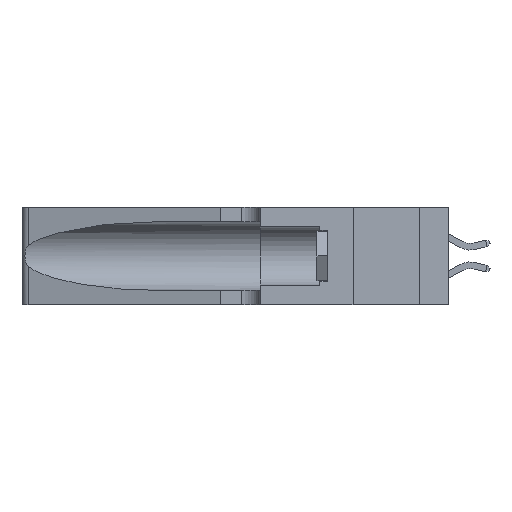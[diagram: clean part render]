
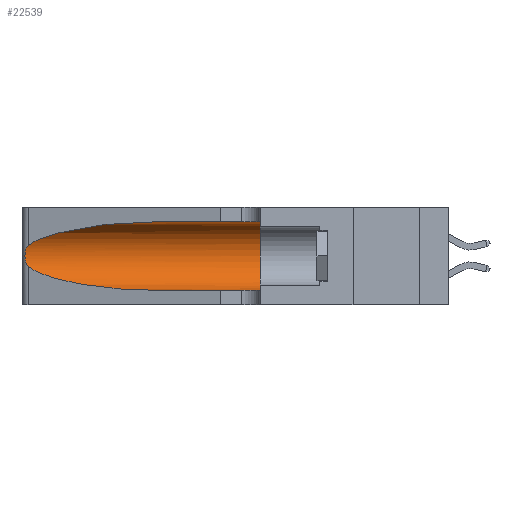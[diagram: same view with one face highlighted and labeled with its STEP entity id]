
A CAD part, left-side view. The second image highlights one B-rep face of the part: STEP entity #22539.
In plain terms, the highlighted cylindrical face has radius 3.308 mm (diameter 6.617 mm), a partial arc.
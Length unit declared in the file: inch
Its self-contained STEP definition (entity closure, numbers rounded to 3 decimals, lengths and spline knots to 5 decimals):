
#822 = AXIS2_PLACEMENT_3D ( 'NONE', #7146, #13845, #24084 ) ;
#1048 = DIRECTION ( 'NONE',  ( 0., -1., 0. ) ) ;
#2286 = CARTESIAN_POINT ( 'NONE',  ( 0.25555, 1.22994, 0.2215 ) ) ;
#2435 = CARTESIAN_POINT ( 'NONE',  ( 0.25854, 1.2359, 0.20912 ) ) ;
#2937 = CARTESIAN_POINT ( 'NONE',  ( 0.1305, 1.61858, 0.31525 ) ) ;
#3580 = VERTEX_POINT ( 'NONE', #40791 ) ;
#3627 = CARTESIAN_POINT ( 'NONE',  ( 0.1305, 0.72297, 0.05475 ) ) ;
#3670 = AXIS2_PLACEMENT_3D ( 'NONE', #38899, #18575, #42254 ) ;
#3993 = EDGE_CURVE ( 'NONE', #22033, #3580, #9045, .T. ) ;
#4248 = VERTEX_POINT ( 'NONE', #3627 ) ;
#5766 =( BOUNDED_CURVE ( )  B_SPLINE_CURVE ( 3, ( #12534, #26208, #9281, #33033 ),
 .UNSPECIFIED., .F., .F. ) 
 B_SPLINE_CURVE_WITH_KNOTS ( ( 4, 4 ),
 ( 3.44316, 4.71239 ),
 .UNSPECIFIED. ) 
 CURVE ( )  GEOMETRIC_REPRESENTATION_ITEM ( )  RATIONAL_B_SPLINE_CURVE ( ( 1., 0.87, 0.87, 1. ) ) 
 REPRESENTATION_ITEM ( '' )  );
#5879 = CARTESIAN_POINT ( 'NONE',  ( 0.26075, 1.23896, 0.19203 ) ) ;
#6364 = DIRECTION ( 'NONE',  ( 0., -1., 0. ) ) ;
#7146 = CARTESIAN_POINT ( 'NONE',  ( 0.1305, 1.61858, 0.185 ) ) ;
#7447 = CIRCLE ( 'NONE', #3670, 0.13025 ) ;
#7490 = ORIENTED_EDGE ( 'NONE', *, *, #11694, .F. ) ;
#7576 = CYLINDRICAL_SURFACE ( 'NONE', #822, 0.13025 ) ;
#8862 = CARTESIAN_POINT ( 'NONE',  ( 0.1305, 0.35, 0.05475 ) ) ;
#9045 = B_SPLINE_CURVE_WITH_KNOTS ( 'NONE', 3,
 ( #36313, #2286, #43065, #22806, #2435, #26228, #5879, #29645, #9307, #33057, #12716, #36456, #16118, #39839 ),
 .UNSPECIFIED., .F., .F.,
 ( 4, 2, 2, 2, 2, 2, 4 ),
 ( 0., 0.00027, 0.00053, 0.00107, 0.0016, 0.00187, 0.00214 ),
 .UNSPECIFIED. ) ;
#9281 = CARTESIAN_POINT ( 'NONE',  ( 0.18966, 0.96281, 0.05475 ) ) ;
#9293 = CARTESIAN_POINT ( 'NONE',  ( 0.18966, 0.96281, 0.31525 ) ) ;
#9307 = CARTESIAN_POINT ( 'NONE',  ( 0.26017, 1.23833, 0.17102 ) ) ;
#11694 = EDGE_CURVE ( 'NONE', #39162, #39043, #23999, .T. ) ;
#11950 = ORIENTED_EDGE ( 'NONE', *, *, #17912, .T. ) ;
#12534 = CARTESIAN_POINT ( 'NONE',  ( 0.25487, 1.22718, 0.14631 ) ) ;
#12716 = CARTESIAN_POINT ( 'NONE',  ( 0.25789, 1.23486, 0.15765 ) ) ;
#13516 = ORIENTED_EDGE ( 'NONE', *, *, #3993, .T. ) ;
#13845 = DIRECTION ( 'NONE',  ( 0., -1., 0. ) ) ;
#14814 = EDGE_CURVE ( 'NONE', #39162, #22033, #21548, .T. ) ;
#16118 = CARTESIAN_POINT ( 'NONE',  ( 0.25555, 1.22993, 0.14849 ) ) ;
#16540 = EDGE_CURVE ( 'NONE', #39043, #33109, #7447, .T. ) ;
#17296 = LINE ( 'NONE', #41724, #34305 ) ;
#17853 = EDGE_LOOP ( 'NONE', ( #41080, #13516, #11950, #31107, #41205, #7490 ) ) ;
#17912 = EDGE_CURVE ( 'NONE', #3580, #4248, #5766, .T. ) ;
#18575 = DIRECTION ( 'NONE',  ( 0., 1., 0. ) ) ;
#19530 = CARTESIAN_POINT ( 'NONE',  ( 0.25487, 1.22718, 0.22369 ) ) ;
#21548 =( BOUNDED_CURVE ( )  B_SPLINE_CURVE ( 3, ( #36437, #9293, #39831, #19530 ),
 .UNSPECIFIED., .F., .F. ) 
 B_SPLINE_CURVE_WITH_KNOTS ( ( 4, 4 ),
 ( 1.5708, 2.84003 ),
 .UNSPECIFIED. ) 
 CURVE ( )  GEOMETRIC_REPRESENTATION_ITEM ( )  RATIONAL_B_SPLINE_CURVE ( ( 1., 0.87, 0.87, 1. ) ) 
 REPRESENTATION_ITEM ( '' )  );
#21874 = CARTESIAN_POINT ( 'NONE',  ( 0.1305, 0.35, 0.31525 ) ) ;
#22033 = VERTEX_POINT ( 'NONE', #38663 ) ;
#22539 = ADVANCED_FACE ( 'NONE', ( #34670 ), #7576, .F. ) ;
#22806 = CARTESIAN_POINT ( 'NONE',  ( 0.25787, 1.23484, 0.2124 ) ) ;
#23999 = LINE ( 'NONE', #2937, #40957 ) ;
#24084 = DIRECTION ( 'NONE',  ( 0., 0., -1. ) ) ;
#26208 = CARTESIAN_POINT ( 'NONE',  ( 0.2373, 1.15595, 0.08982 ) ) ;
#26228 = CARTESIAN_POINT ( 'NONE',  ( 0.26018, 1.23835, 0.19895 ) ) ;
#29645 = CARTESIAN_POINT ( 'NONE',  ( 0.26075, 1.23896, 0.178 ) ) ;
#31107 = ORIENTED_EDGE ( 'NONE', *, *, #38966, .T. ) ;
#33033 = CARTESIAN_POINT ( 'NONE',  ( 0.1305, 0.72297, 0.05475 ) ) ;
#33057 = CARTESIAN_POINT ( 'NONE',  ( 0.25856, 1.23593, 0.16098 ) ) ;
#33109 = VERTEX_POINT ( 'NONE', #8862 ) ;
#34305 = VECTOR ( 'NONE', #1048, 39.37008 ) ;
#34670 = FACE_OUTER_BOUND ( 'NONE', #17853, .T. ) ;
#35813 = CARTESIAN_POINT ( 'NONE',  ( 0.1305, 0.72297, 0.31525 ) ) ;
#36313 = CARTESIAN_POINT ( 'NONE',  ( 0.25487, 1.22718, 0.22369 ) ) ;
#36437 = CARTESIAN_POINT ( 'NONE',  ( 0.1305, 0.72297, 0.31525 ) ) ;
#36456 = CARTESIAN_POINT ( 'NONE',  ( 0.25639, 1.23186, 0.15144 ) ) ;
#38663 = CARTESIAN_POINT ( 'NONE',  ( 0.25487, 1.22718, 0.22369 ) ) ;
#38899 = CARTESIAN_POINT ( 'NONE',  ( 0.1305, 0.35, 0.185 ) ) ;
#38966 = EDGE_CURVE ( 'NONE', #4248, #33109, #17296, .T. ) ;
#39043 = VERTEX_POINT ( 'NONE', #21874 ) ;
#39162 = VERTEX_POINT ( 'NONE', #35813 ) ;
#39831 = CARTESIAN_POINT ( 'NONE',  ( 0.2373, 1.15595, 0.28018 ) ) ;
#39839 = CARTESIAN_POINT ( 'NONE',  ( 0.25487, 1.22718, 0.14631 ) ) ;
#40791 = CARTESIAN_POINT ( 'NONE',  ( 0.25487, 1.22718, 0.14631 ) ) ;
#40957 = VECTOR ( 'NONE', #6364, 39.37008 ) ;
#41080 = ORIENTED_EDGE ( 'NONE', *, *, #14814, .T. ) ;
#41205 = ORIENTED_EDGE ( 'NONE', *, *, #16540, .F. ) ;
#41724 = CARTESIAN_POINT ( 'NONE',  ( 0.1305, 1.61858, 0.05475 ) ) ;
#42254 = DIRECTION ( 'NONE',  ( 0., 0., 1. ) ) ;
#43065 = CARTESIAN_POINT ( 'NONE',  ( 0.25639, 1.23184, 0.21858 ) ) ;
